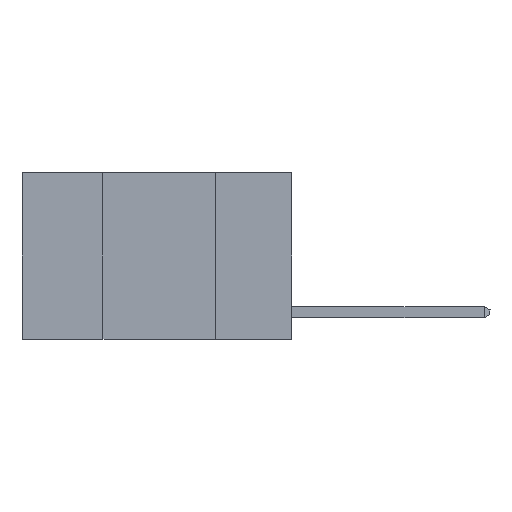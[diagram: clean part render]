
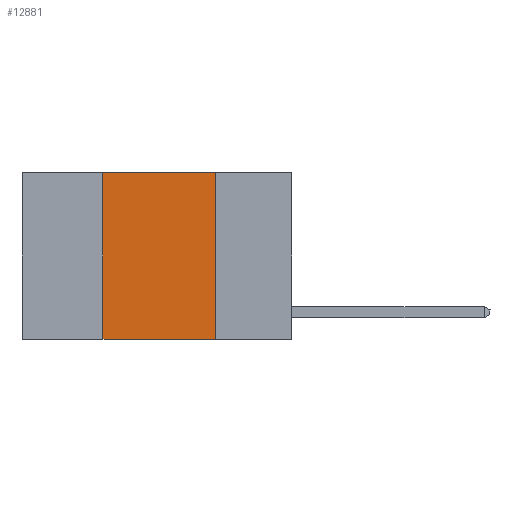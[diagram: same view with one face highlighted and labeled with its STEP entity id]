
A CAD part, left-side view. The second image highlights one B-rep face of the part: STEP entity #12881.
In plain terms, the highlighted planar face has unit normal (-1, 0, 0).
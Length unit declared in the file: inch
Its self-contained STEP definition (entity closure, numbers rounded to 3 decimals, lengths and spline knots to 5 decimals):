
#1902 = FACE_OUTER_BOUND ( 'NONE', #21085, .T. ) ;
#2495 = VERTEX_POINT ( 'NONE', #19958 ) ;
#3454 = EDGE_CURVE ( 'NONE', #3532, #22632, #27708, .T. ) ;
#3532 = VERTEX_POINT ( 'NONE', #16688 ) ;
#3640 = VERTEX_POINT ( 'NONE', #16977 ) ;
#4604 = EDGE_CURVE ( 'NONE', #2495, #22632, #24159, .T. ) ;
#5859 = EDGE_CURVE ( 'NONE', #3532, #3640, #15519, .T. ) ;
#6251 = VECTOR ( 'NONE', #6424, 39.37008 ) ;
#6424 = DIRECTION ( 'NONE',  ( 0., 0., -1. ) ) ;
#8785 = CARTESIAN_POINT ( 'NONE',  ( 0., 0.17, -0.37 ) ) ;
#8861 = CARTESIAN_POINT ( 'NONE',  ( 0., 0.6, 0. ) ) ;
#9481 = ORIENTED_EDGE ( 'NONE', *, *, #12724, .F. ) ;
#9623 = ORIENTED_EDGE ( 'NONE', *, *, #5859, .F. ) ;
#10376 = CARTESIAN_POINT ( 'NONE',  ( 0., 0.6, 0. ) ) ;
#11121 = PLANE ( 'NONE',  #13719 ) ;
#11282 = VECTOR ( 'NONE', #28793, 39.37008 ) ;
#12724 = EDGE_CURVE ( 'NONE', #3640, #2495, #19596, .T. ) ;
#12881 = ADVANCED_FACE ( 'NONE', ( #1902 ), #11121, .F. ) ;
#13719 = AXIS2_PLACEMENT_3D ( 'NONE', #8861, #20336, #29545 ) ;
#15223 = DIRECTION ( 'NONE',  ( 0., 0., 1. ) ) ;
#15519 = LINE ( 'NONE', #28964, #24690 ) ;
#16688 = CARTESIAN_POINT ( 'NONE',  ( 0., 0.42, -0.37 ) ) ;
#16977 = CARTESIAN_POINT ( 'NONE',  ( 0., 0.42, 0. ) ) ;
#18340 = DIRECTION ( 'NONE',  ( 0., -1., 0. ) ) ;
#19596 = LINE ( 'NONE', #10376, #11282 ) ;
#19958 = CARTESIAN_POINT ( 'NONE',  ( 0., 0.17, 0. ) ) ;
#20336 = DIRECTION ( 'NONE',  ( 1., 0., 0. ) ) ;
#21085 = EDGE_LOOP ( 'NONE', ( #27275, #9481, #9623, #22900 ) ) ;
#22154 = VECTOR ( 'NONE', #18340, 39.37008 ) ;
#22632 = VERTEX_POINT ( 'NONE', #8785 ) ;
#22900 = ORIENTED_EDGE ( 'NONE', *, *, #3454, .T. ) ;
#24159 = LINE ( 'NONE', #28080, #6251 ) ;
#24690 = VECTOR ( 'NONE', #15223, 39.37008 ) ;
#27275 = ORIENTED_EDGE ( 'NONE', *, *, #4604, .F. ) ;
#27708 = LINE ( 'NONE', #27851, #22154 ) ;
#27851 = CARTESIAN_POINT ( 'NONE',  ( 0., 0.6, -0.37 ) ) ;
#28080 = CARTESIAN_POINT ( 'NONE',  ( 0., 0.17, 0. ) ) ;
#28793 = DIRECTION ( 'NONE',  ( 0., -1., 0. ) ) ;
#28964 = CARTESIAN_POINT ( 'NONE',  ( 0., 0.42, 0. ) ) ;
#29545 = DIRECTION ( 'NONE',  ( 0., 0., -1. ) ) ;
